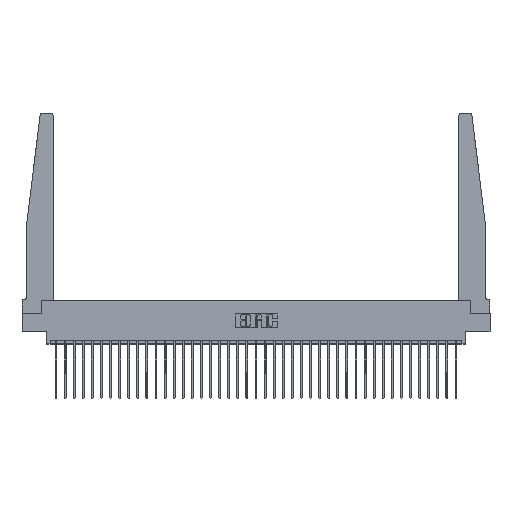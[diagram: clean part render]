
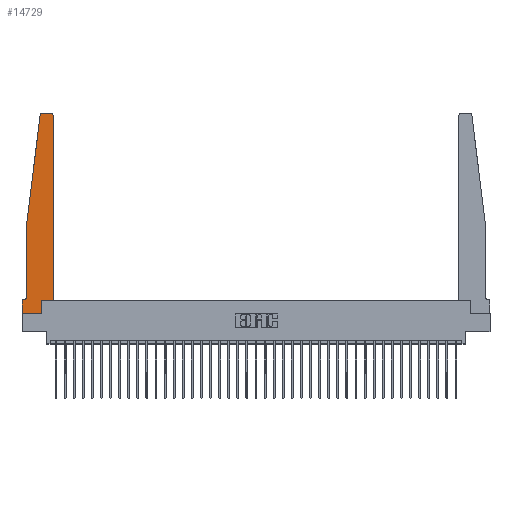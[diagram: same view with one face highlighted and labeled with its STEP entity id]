
A CAD part, top view. The second image highlights one B-rep face of the part: STEP entity #14729.
In plain terms, the highlighted planar face has unit normal (0, 0, 1).
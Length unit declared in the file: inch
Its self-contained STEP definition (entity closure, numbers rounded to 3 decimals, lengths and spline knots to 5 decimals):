
#596 = ORIENTED_EDGE ( 'NONE', *, *, #7855, .T. ) ;
#1941 = VERTEX_POINT ( 'NONE', #12101 ) ;
#2013 = DIRECTION ( 'NONE',  ( 1., 0., 0. ) ) ;
#2546 = LINE ( 'NONE', #23021, #30900 ) ;
#2645 = CARTESIAN_POINT ( 'NONE',  ( 0.015, 0.2375, 0.37 ) ) ;
#2749 = CARTESIAN_POINT ( 'NONE',  ( 0.425, 0.18, 0.37 ) ) ;
#2778 = VERTEX_POINT ( 'NONE', #4538 ) ;
#2937 = VECTOR ( 'NONE', #13975, 39.37008 ) ;
#3154 = DIRECTION ( 'NONE',  ( 0., 0., -1. ) ) ;
#3255 = EDGE_CURVE ( 'NONE', #2778, #25884, #2546, .T. ) ;
#3283 = CARTESIAN_POINT ( 'NONE',  ( 0.425, 0.18, 0.37 ) ) ;
#3600 = LINE ( 'NONE', #22348, #23264 ) ;
#3686 = VECTOR ( 'NONE', #14082, 39.37008 ) ;
#3841 = ORIENTED_EDGE ( 'NONE', *, *, #3255, .T. ) ;
#4256 = EDGE_CURVE ( 'NONE', #24137, #1941, #28396, .T. ) ;
#4274 = VECTOR ( 'NONE', #20494, 39.37008 ) ;
#4446 = VERTEX_POINT ( 'NONE', #33525 ) ;
#4538 = CARTESIAN_POINT ( 'NONE',  ( 0., 0., 0.37 ) ) ;
#4770 = EDGE_CURVE ( 'NONE', #7421, #23447, #11616, .T. ) ;
#5142 = DIRECTION ( 'NONE',  ( 0., -1., 0. ) ) ;
#5195 = DIRECTION ( 'NONE',  ( 1., 0., 0. ) ) ;
#5432 = DIRECTION ( 'NONE',  ( -1., 0., 0. ) ) ;
#5682 = VERTEX_POINT ( 'NONE', #34302 ) ;
#5721 = CARTESIAN_POINT ( 'NONE',  ( 0.24675, 2.72367, 0.37 ) ) ;
#5858 = CARTESIAN_POINT ( 'NONE',  ( 0.425, 2.72, 0.37 ) ) ;
#6670 = ORIENTED_EDGE ( 'NONE', *, *, #25572, .T. ) ;
#6681 = ORIENTED_EDGE ( 'NONE', *, *, #4256, .T. ) ;
#7011 = CARTESIAN_POINT ( 'NONE',  ( 0.065, 1.25, 0.37 ) ) ;
#7139 = CARTESIAN_POINT ( 'NONE',  ( 0.2605, 0.18, 0.37 ) ) ;
#7386 = VERTEX_POINT ( 'NONE', #7011 ) ;
#7421 = VERTEX_POINT ( 'NONE', #18450 ) ;
#7626 = CIRCLE ( 'NONE', #28147, 0.03 ) ;
#7855 = EDGE_CURVE ( 'NONE', #25884, #7421, #12505, .T. ) ;
#7959 = DIRECTION ( 'NONE',  ( 1., 0., 0. ) ) ;
#8282 = CARTESIAN_POINT ( 'NONE',  ( 0.2605, 0., 0.37 ) ) ;
#8538 = EDGE_LOOP ( 'NONE', ( #27378, #22828, #13271, #28745, #6681, #6670, #28277, #3841, #596, #21676, #20934, #33975 ) ) ;
#9882 = EDGE_CURVE ( 'NONE', #9964, #7386, #3600, .T. ) ;
#9964 = VERTEX_POINT ( 'NONE', #5721 ) ;
#11616 = LINE ( 'NONE', #3283, #24385 ) ;
#11621 = VERTEX_POINT ( 'NONE', #5858 ) ;
#11808 = CARTESIAN_POINT ( 'NONE',  ( 0.25, 2.75, 0.37 ) ) ;
#12098 = DIRECTION ( 'NONE',  ( -1., 0., 0. ) ) ;
#12101 = CARTESIAN_POINT ( 'NONE',  ( 0.015, 0.1875, 0.37 ) ) ;
#12505 = LINE ( 'NONE', #7139, #4274 ) ;
#13271 = ORIENTED_EDGE ( 'NONE', *, *, #9882, .T. ) ;
#13433 = AXIS2_PLACEMENT_3D ( 'NONE', #2645, #3154, #5432 ) ;
#13466 = EDGE_CURVE ( 'NONE', #4446, #2778, #19190, .T. ) ;
#13858 = DIRECTION ( 'NONE',  ( 0., 1., 0. ) ) ;
#13975 = DIRECTION ( 'NONE',  ( 0., -1., 0. ) ) ;
#14082 = DIRECTION ( 'NONE',  ( -1., 0., 0. ) ) ;
#14527 = LINE ( 'NONE', #20251, #15511 ) ;
#14729 = ADVANCED_FACE ( 'NONE', ( #18855 ), #31545, .T. ) ;
#14898 = CARTESIAN_POINT ( 'NONE',  ( 0.27653, 2.75, 0.37 ) ) ;
#15511 = VECTOR ( 'NONE', #12098, 39.37008 ) ;
#15763 = VERTEX_POINT ( 'NONE', #14898 ) ;
#15822 = CARTESIAN_POINT ( 'NONE',  ( 0.425, 0.18, 0.37 ) ) ;
#15947 = CARTESIAN_POINT ( 'NONE',  ( 0.27653, 2.72, 0.37 ) ) ;
#16120 = EDGE_CURVE ( 'NONE', #23447, #11621, #27064, .T. ) ;
#16481 = DIRECTION ( 'NONE',  ( -0.122, -0.992, 0. ) ) ;
#17302 = EDGE_CURVE ( 'NONE', #15763, #9964, #20202, .T. ) ;
#18450 = CARTESIAN_POINT ( 'NONE',  ( 0.2605, 0.18, 0.37 ) ) ;
#18570 = CARTESIAN_POINT ( 'NONE',  ( 0.395, 2.72, 0.37 ) ) ;
#18850 = VECTOR ( 'NONE', #5142, 39.37008 ) ;
#18855 = FACE_OUTER_BOUND ( 'NONE', #8538, .T. ) ;
#19162 = VECTOR ( 'NONE', #13858, 39.37008 ) ;
#19190 = LINE ( 'NONE', #29796, #2937 ) ;
#19244 = CARTESIAN_POINT ( 'NONE',  ( 0.065, 0.2375, 0.37 ) ) ;
#19973 = LINE ( 'NONE', #11808, #3686 ) ;
#20202 = CIRCLE ( 'NONE', #30217, 0.03 ) ;
#20251 = CARTESIAN_POINT ( 'NONE',  ( 0.065, 0.1875, 0.37 ) ) ;
#20372 = EDGE_CURVE ( 'NONE', #5682, #15763, #19973, .T. ) ;
#20494 = DIRECTION ( 'NONE',  ( 0., 1., 0. ) ) ;
#20688 = EDGE_CURVE ( 'NONE', #11621, #5682, #7626, .T. ) ;
#20934 = ORIENTED_EDGE ( 'NONE', *, *, #16120, .T. ) ;
#21676 = ORIENTED_EDGE ( 'NONE', *, *, #4770, .T. ) ;
#22348 = CARTESIAN_POINT ( 'NONE',  ( 0.065, 1.25, 0.37 ) ) ;
#22828 = ORIENTED_EDGE ( 'NONE', *, *, #17302, .T. ) ;
#23021 = CARTESIAN_POINT ( 'NONE',  ( 0., 0., 0.37 ) ) ;
#23191 = CARTESIAN_POINT ( 'NONE',  ( 0.065, 1.25, 0.37 ) ) ;
#23264 = VECTOR ( 'NONE', #16481, 39.37008 ) ;
#23447 = VERTEX_POINT ( 'NONE', #15822 ) ;
#24137 = VERTEX_POINT ( 'NONE', #19244 ) ;
#24385 = VECTOR ( 'NONE', #29703, 39.37008 ) ;
#25572 = EDGE_CURVE ( 'NONE', #1941, #4446, #14527, .T. ) ;
#25821 = EDGE_CURVE ( 'NONE', #7386, #24137, #33976, .T. ) ;
#25884 = VERTEX_POINT ( 'NONE', #8282 ) ;
#26312 = DIRECTION ( 'NONE',  ( 0., 0., 1. ) ) ;
#27064 = LINE ( 'NONE', #2749, #19162 ) ;
#27378 = ORIENTED_EDGE ( 'NONE', *, *, #20372, .T. ) ;
#28147 = AXIS2_PLACEMENT_3D ( 'NONE', #18570, #32152, #5195 ) ;
#28277 = ORIENTED_EDGE ( 'NONE', *, *, #13466, .T. ) ;
#28396 = CIRCLE ( 'NONE', #13433, 0.05 ) ;
#28745 = ORIENTED_EDGE ( 'NONE', *, *, #25821, .T. ) ;
#29462 = CARTESIAN_POINT ( 'NONE',  ( 0., 0.1875, 0.37 ) ) ;
#29703 = DIRECTION ( 'NONE',  ( 1., 0., 0. ) ) ;
#29796 = CARTESIAN_POINT ( 'NONE',  ( 0., 0., 0.37 ) ) ;
#30217 = AXIS2_PLACEMENT_3D ( 'NONE', #15947, #31772, #7959 ) ;
#30900 = VECTOR ( 'NONE', #2013, 39.37008 ) ;
#31545 = PLANE ( 'NONE',  #31849 ) ;
#31772 = DIRECTION ( 'NONE',  ( 0., 0., 1. ) ) ;
#31849 = AXIS2_PLACEMENT_3D ( 'NONE', #29462, #26312, #34309 ) ;
#32152 = DIRECTION ( 'NONE',  ( 0., 0., 1. ) ) ;
#33525 = CARTESIAN_POINT ( 'NONE',  ( 0., 0.1875, 0.37 ) ) ;
#33975 = ORIENTED_EDGE ( 'NONE', *, *, #20688, .T. ) ;
#33976 = LINE ( 'NONE', #23191, #18850 ) ;
#34302 = CARTESIAN_POINT ( 'NONE',  ( 0.395, 2.75, 0.37 ) ) ;
#34309 = DIRECTION ( 'NONE',  ( 1., 0., 0. ) ) ;
